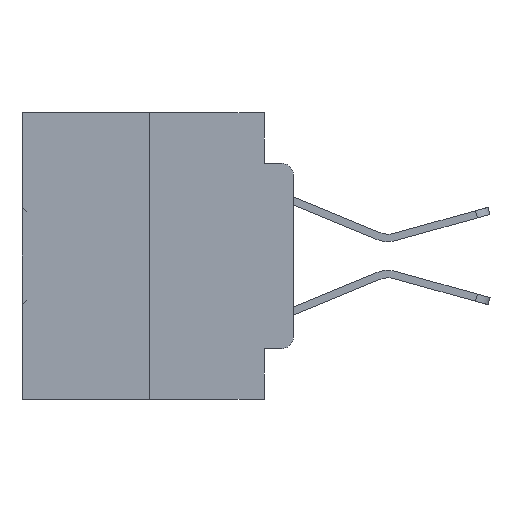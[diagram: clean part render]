
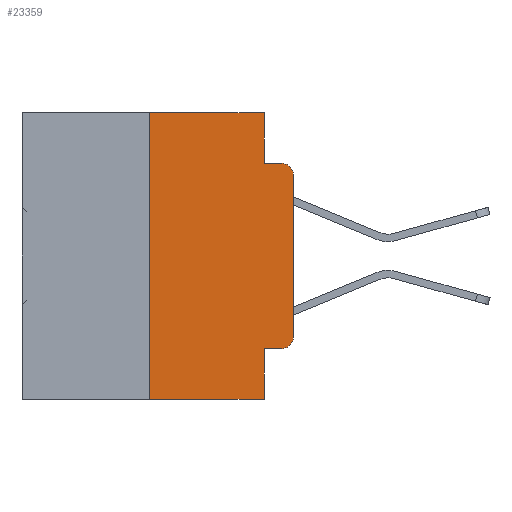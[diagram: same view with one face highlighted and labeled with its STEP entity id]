
A CAD part, left-side view. The second image highlights one B-rep face of the part: STEP entity #23359.
In plain terms, the highlighted planar face has unit normal (-1, 0, 0).
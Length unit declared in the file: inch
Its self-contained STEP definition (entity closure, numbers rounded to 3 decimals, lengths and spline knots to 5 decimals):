
#261 = ORIENTED_EDGE ( 'NONE', *, *, #12271, .F. ) ;
#415 = VECTOR ( 'NONE', #30414, 39.37008 ) ;
#488 = ORIENTED_EDGE ( 'NONE', *, *, #8630, .F. ) ;
#522 = DIRECTION ( 'NONE',  ( 0., 0., -1. ) ) ;
#978 = EDGE_LOOP ( 'NONE', ( #9192, #20732, #261, #17199, #33946, #4650, #22064, #488, #29087, #37096 ) ) ;
#1238 = CARTESIAN_POINT ( 'NONE',  ( 0., 0.473, 0. ) ) ;
#2002 = DIRECTION ( 'NONE',  ( 0., 0., -1. ) ) ;
#3458 = VERTEX_POINT ( 'NONE', #15978 ) ;
#4650 = ORIENTED_EDGE ( 'NONE', *, *, #14874, .F. ) ;
#4825 = VERTEX_POINT ( 'NONE', #11071 ) ;
#5681 = VERTEX_POINT ( 'NONE', #6452 ) ;
#5969 = VECTOR ( 'NONE', #27133, 39.37008 ) ;
#6387 = VECTOR ( 'NONE', #35196, 39.37008 ) ;
#6452 = CARTESIAN_POINT ( 'NONE',  ( 0., 0.02, -0.4115 ) ) ;
#6761 = LINE ( 'NONE', #26587, #36384 ) ;
#7017 = CARTESIAN_POINT ( 'NONE',  ( 0., 0.473, -0.5 ) ) ;
#8185 = LINE ( 'NONE', #28323, #20767 ) ;
#8225 = LINE ( 'NONE', #7017, #5969 ) ;
#8232 = CARTESIAN_POINT ( 'NONE',  ( 0., 0.051, -0.4115 ) ) ;
#8630 = EDGE_CURVE ( 'NONE', #21633, #11537, #6761, .T. ) ;
#8700 = VECTOR ( 'NONE', #36383, 39.37008 ) ;
#8779 = EDGE_CURVE ( 'NONE', #21633, #5681, #12632, .T. ) ;
#9192 = ORIENTED_EDGE ( 'NONE', *, *, #26168, .T. ) ;
#9824 = DIRECTION ( 'NONE',  ( -1., 0., 0. ) ) ;
#10426 = EDGE_CURVE ( 'NONE', #29159, #24936, #13376, .T. ) ;
#10862 = CARTESIAN_POINT ( 'NONE',  ( 0., 0.051, -0.0885 ) ) ;
#11071 = CARTESIAN_POINT ( 'NONE',  ( 0., 0.25, -0.5 ) ) ;
#11537 = VERTEX_POINT ( 'NONE', #32696 ) ;
#12271 = EDGE_CURVE ( 'NONE', #25361, #24936, #15967, .T. ) ;
#12632 = LINE ( 'NONE', #15707, #32375 ) ;
#12671 = PLANE ( 'NONE',  #22423 ) ;
#12723 = DIRECTION ( 'NONE',  ( 0., 0., -1. ) ) ;
#13005 = CARTESIAN_POINT ( 'NONE',  ( 0., 0.25, 0. ) ) ;
#13135 = CARTESIAN_POINT ( 'NONE',  ( 0., 0., -0.3915 ) ) ;
#13376 = CIRCLE ( 'NONE', #32872, 0.02 ) ;
#13484 = CARTESIAN_POINT ( 'NONE',  ( 0., 0.051, -0.0885 ) ) ;
#13661 = DIRECTION ( 'NONE',  ( 0., 0., 1. ) ) ;
#13861 = CARTESIAN_POINT ( 'NONE',  ( 0., 0.02, -0.0885 ) ) ;
#14874 = EDGE_CURVE ( 'NONE', #4825, #25569, #8185, .T. ) ;
#14923 = DIRECTION ( 'NONE',  ( 0., 0., -1. ) ) ;
#15172 = CARTESIAN_POINT ( 'NONE',  ( 0., 0.051, 0. ) ) ;
#15515 = CARTESIAN_POINT ( 'NONE',  ( 0., 0.02, -0.1085 ) ) ;
#15707 = CARTESIAN_POINT ( 'NONE',  ( 0., 0.051, -0.4115 ) ) ;
#15967 = LINE ( 'NONE', #13484, #8700 ) ;
#15978 = CARTESIAN_POINT ( 'NONE',  ( 0., 0.051, 0. ) ) ;
#16370 = DIRECTION ( 'NONE',  ( 1., 0., 0. ) ) ;
#17199 = ORIENTED_EDGE ( 'NONE', *, *, #23775, .F. ) ;
#17799 = CARTESIAN_POINT ( 'NONE',  ( 0., 0.02, -0.3915 ) ) ;
#19085 = AXIS2_PLACEMENT_3D ( 'NONE', #17799, #32275, #522 ) ;
#20208 = CARTESIAN_POINT ( 'NONE',  ( 0., 0.473, 0. ) ) ;
#20732 = ORIENTED_EDGE ( 'NONE', *, *, #10426, .T. ) ;
#20767 = VECTOR ( 'NONE', #13661, 39.37008 ) ;
#20806 = DIRECTION ( 'NONE',  ( 0., -1., 0. ) ) ;
#21633 = VERTEX_POINT ( 'NONE', #8232 ) ;
#22064 = ORIENTED_EDGE ( 'NONE', *, *, #36094, .T. ) ;
#22423 = AXIS2_PLACEMENT_3D ( 'NONE', #1238, #16370, #2002 ) ;
#23005 = CIRCLE ( 'NONE', #19085, 0.02 ) ;
#23359 = ADVANCED_FACE ( 'NONE', ( #31578 ), #12671, .F. ) ;
#23626 = EDGE_CURVE ( 'NONE', #25569, #3458, #32009, .T. ) ;
#23775 = EDGE_CURVE ( 'NONE', #3458, #25361, #33827, .T. ) ;
#24015 = CARTESIAN_POINT ( 'NONE',  ( 0., 0., 0. ) ) ;
#24322 = DIRECTION ( 'NONE',  ( 0., -1., 0. ) ) ;
#24421 = EDGE_CURVE ( 'NONE', #5681, #34968, #23005, .T. ) ;
#24936 = VERTEX_POINT ( 'NONE', #13861 ) ;
#25361 = VERTEX_POINT ( 'NONE', #10862 ) ;
#25569 = VERTEX_POINT ( 'NONE', #13005 ) ;
#26168 = EDGE_CURVE ( 'NONE', #34968, #29159, #34113, .T. ) ;
#26587 = CARTESIAN_POINT ( 'NONE',  ( 0., 0.051, 0. ) ) ;
#27133 = DIRECTION ( 'NONE',  ( 0., -1., 0. ) ) ;
#28323 = CARTESIAN_POINT ( 'NONE',  ( 0., 0.25, 0. ) ) ;
#29087 = ORIENTED_EDGE ( 'NONE', *, *, #8779, .T. ) ;
#29159 = VERTEX_POINT ( 'NONE', #31868 ) ;
#30414 = DIRECTION ( 'NONE',  ( 0., 0., 1. ) ) ;
#31130 = VECTOR ( 'NONE', #20806, 39.37008 ) ;
#31578 = FACE_OUTER_BOUND ( 'NONE', #978, .T. ) ;
#31868 = CARTESIAN_POINT ( 'NONE',  ( 0., 0., -0.1085 ) ) ;
#32009 = LINE ( 'NONE', #20208, #31130 ) ;
#32275 = DIRECTION ( 'NONE',  ( -1., 0., 0. ) ) ;
#32375 = VECTOR ( 'NONE', #24322, 39.37008 ) ;
#32696 = CARTESIAN_POINT ( 'NONE',  ( 0., 0.051, -0.5 ) ) ;
#32872 = AXIS2_PLACEMENT_3D ( 'NONE', #15515, #9824, #12723 ) ;
#33827 = LINE ( 'NONE', #15172, #6387 ) ;
#33946 = ORIENTED_EDGE ( 'NONE', *, *, #23626, .F. ) ;
#34113 = LINE ( 'NONE', #24015, #415 ) ;
#34968 = VERTEX_POINT ( 'NONE', #13135 ) ;
#35196 = DIRECTION ( 'NONE',  ( 0., 0., -1. ) ) ;
#36094 = EDGE_CURVE ( 'NONE', #4825, #11537, #8225, .T. ) ;
#36383 = DIRECTION ( 'NONE',  ( 0., -1., 0. ) ) ;
#36384 = VECTOR ( 'NONE', #14923, 39.37008 ) ;
#37096 = ORIENTED_EDGE ( 'NONE', *, *, #24421, .T. ) ;
